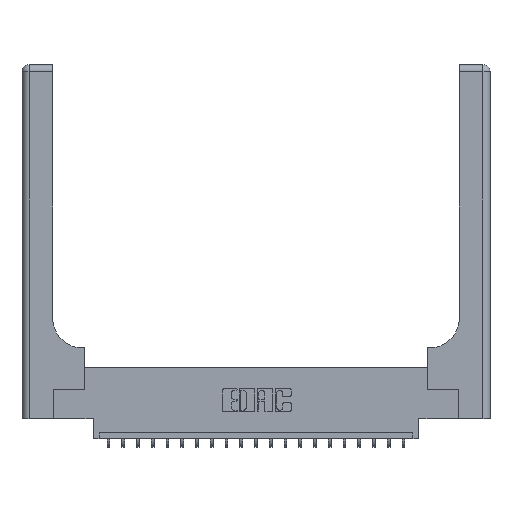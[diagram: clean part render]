
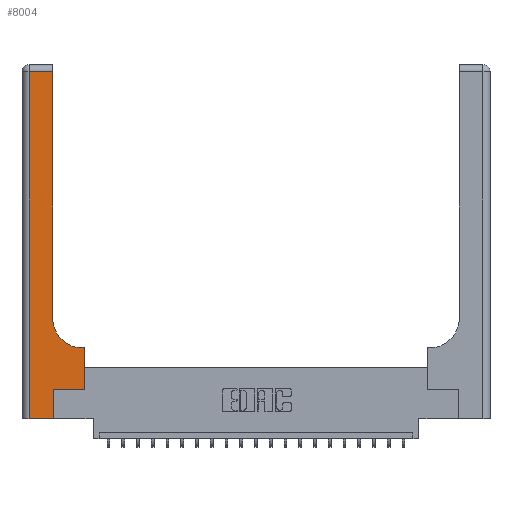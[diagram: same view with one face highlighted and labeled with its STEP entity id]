
A CAD part, top view. The second image highlights one B-rep face of the part: STEP entity #8004.
In plain terms, the highlighted planar face has unit normal (0, 0, 1).
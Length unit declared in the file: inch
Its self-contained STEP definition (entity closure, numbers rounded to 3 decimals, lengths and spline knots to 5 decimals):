
#139 = DIRECTION ( 'NONE',  ( 1., 0., 0. ) ) ;
#195 = VERTEX_POINT ( 'NONE', #5237 ) ;
#292 = ORIENTED_EDGE ( 'NONE', *, *, #7281, .T. ) ;
#694 = VECTOR ( 'NONE', #3284, 39.37008 ) ;
#792 = LINE ( 'NONE', #9459, #17234 ) ;
#831 = DIRECTION ( 'NONE',  ( 0., 1., 0. ) ) ;
#1504 = EDGE_CURVE ( 'NONE', #2372, #5062, #1699, .T. ) ;
#1699 = LINE ( 'NONE', #9031, #18096 ) ;
#1843 = CARTESIAN_POINT ( 'NONE',  ( 0., 0., 0.37 ) ) ;
#1953 = ORIENTED_EDGE ( 'NONE', *, *, #10798, .T. ) ;
#2227 = VECTOR ( 'NONE', #15557, 39.37008 ) ;
#2372 = VERTEX_POINT ( 'NONE', #16083 ) ;
#3246 = CARTESIAN_POINT ( 'NONE',  ( 0.265, 0., 0.37 ) ) ;
#3284 = DIRECTION ( 'NONE',  ( -1., 0., 0. ) ) ;
#3548 = AXIS2_PLACEMENT_3D ( 'NONE', #13962, #5789, #17233 ) ;
#3799 = LINE ( 'NONE', #13714, #11965 ) ;
#4118 = CARTESIAN_POINT ( 'NONE',  ( 0.265, 0.25, 0.37 ) ) ;
#5062 = VERTEX_POINT ( 'NONE', #11935 ) ;
#5063 = CARTESIAN_POINT ( 'NONE',  ( 0.265, 0., 0.37 ) ) ;
#5109 = LINE ( 'NONE', #13099, #694 ) ;
#5237 = CARTESIAN_POINT ( 'NONE',  ( 0.26, 2.94, 0.37 ) ) ;
#5389 = CARTESIAN_POINT ( 'NONE',  ( 0.06, 3., 0.37 ) ) ;
#5470 = ORIENTED_EDGE ( 'NONE', *, *, #7007, .T. ) ;
#5528 = DIRECTION ( 'NONE',  ( 0., 1., 0. ) ) ;
#5789 = DIRECTION ( 'NONE',  ( 0., 0., -1. ) ) ;
#6094 = VERTEX_POINT ( 'NONE', #11863 ) ;
#6706 = DIRECTION ( 'NONE',  ( 0., 1., 0. ) ) ;
#6985 = ORIENTED_EDGE ( 'NONE', *, *, #1504, .T. ) ;
#7007 = EDGE_CURVE ( 'NONE', #5062, #9812, #792, .T. ) ;
#7031 = DIRECTION ( 'NONE',  ( 0., -1., 0. ) ) ;
#7090 = LINE ( 'NONE', #4118, #2227 ) ;
#7281 = EDGE_CURVE ( 'NONE', #6094, #13573, #13150, .T. ) ;
#8004 = ADVANCED_FACE ( 'NONE', ( #15421 ), #18783, .F. ) ;
#9031 = CARTESIAN_POINT ( 'NONE',  ( 0.528, 0.25, 0.37 ) ) ;
#9459 = CARTESIAN_POINT ( 'NONE',  ( 0.26, 0.6, 0.37 ) ) ;
#9812 = VERTEX_POINT ( 'NONE', #17151 ) ;
#9993 = DIRECTION ( 'NONE',  ( 0., 0., -1. ) ) ;
#10012 = EDGE_CURVE ( 'NONE', #195, #6094, #5109, .T. ) ;
#10102 = EDGE_CURVE ( 'NONE', #13257, #14420, #20461, .T. ) ;
#10221 = ORIENTED_EDGE ( 'NONE', *, *, #14372, .T. ) ;
#10798 = EDGE_CURVE ( 'NONE', #16627, #195, #3799, .T. ) ;
#10967 = AXIS2_PLACEMENT_3D ( 'NONE', #19806, #9993, #139 ) ;
#11196 = CARTESIAN_POINT ( 'NONE',  ( 0.26, 0.85, 0.37 ) ) ;
#11824 = EDGE_LOOP ( 'NONE', ( #1953, #14927, #292, #10221, #21169, #12313, #6985, #5470, #13482 ) ) ;
#11863 = CARTESIAN_POINT ( 'NONE',  ( 0.06, 2.94, 0.37 ) ) ;
#11935 = CARTESIAN_POINT ( 'NONE',  ( 0.528, 0.6, 0.37 ) ) ;
#11965 = VECTOR ( 'NONE', #5528, 39.37008 ) ;
#12235 = EDGE_CURVE ( 'NONE', #9812, #16627, #17306, .T. ) ;
#12313 = ORIENTED_EDGE ( 'NONE', *, *, #19527, .T. ) ;
#13099 = CARTESIAN_POINT ( 'NONE',  ( 0., 2.94, 0.37 ) ) ;
#13150 = LINE ( 'NONE', #5389, #16448 ) ;
#13257 = VERTEX_POINT ( 'NONE', #3246 ) ;
#13471 = CARTESIAN_POINT ( 'NONE',  ( 0.265, 0.25, 0.37 ) ) ;
#13482 = ORIENTED_EDGE ( 'NONE', *, *, #12235, .T. ) ;
#13573 = VERTEX_POINT ( 'NONE', #15384 ) ;
#13714 = CARTESIAN_POINT ( 'NONE',  ( 0.26, 3., 0.37 ) ) ;
#13886 = VECTOR ( 'NONE', #18091, 39.37008 ) ;
#13962 = CARTESIAN_POINT ( 'NONE',  ( 0., 3., 0.37 ) ) ;
#14372 = EDGE_CURVE ( 'NONE', #13573, #13257, #18212, .T. ) ;
#14420 = VERTEX_POINT ( 'NONE', #13471 ) ;
#14927 = ORIENTED_EDGE ( 'NONE', *, *, #10012, .T. ) ;
#15384 = CARTESIAN_POINT ( 'NONE',  ( 0.06, 0., 0.37 ) ) ;
#15421 = FACE_OUTER_BOUND ( 'NONE', #11824, .T. ) ;
#15557 = DIRECTION ( 'NONE',  ( 1., 0., 0. ) ) ;
#16083 = CARTESIAN_POINT ( 'NONE',  ( 0.528, 0.25, 0.37 ) ) ;
#16121 = DIRECTION ( 'NONE',  ( -1., 0., 0. ) ) ;
#16448 = VECTOR ( 'NONE', #7031, 39.37008 ) ;
#16627 = VERTEX_POINT ( 'NONE', #11196 ) ;
#17151 = CARTESIAN_POINT ( 'NONE',  ( 0.51, 0.6, 0.37 ) ) ;
#17233 = DIRECTION ( 'NONE',  ( -1., 0., 0. ) ) ;
#17234 = VECTOR ( 'NONE', #16121, 39.37008 ) ;
#17306 = CIRCLE ( 'NONE', #10967, 0.25 ) ;
#17640 = VECTOR ( 'NONE', #6706, 39.37008 ) ;
#18091 = DIRECTION ( 'NONE',  ( 1., 0., 0. ) ) ;
#18096 = VECTOR ( 'NONE', #831, 39.37008 ) ;
#18212 = LINE ( 'NONE', #1843, #13886 ) ;
#18783 = PLANE ( 'NONE',  #3548 ) ;
#19527 = EDGE_CURVE ( 'NONE', #14420, #2372, #7090, .T. ) ;
#19806 = CARTESIAN_POINT ( 'NONE',  ( 0.51, 0.85, 0.37 ) ) ;
#20461 = LINE ( 'NONE', #5063, #17640 ) ;
#21169 = ORIENTED_EDGE ( 'NONE', *, *, #10102, .T. ) ;
